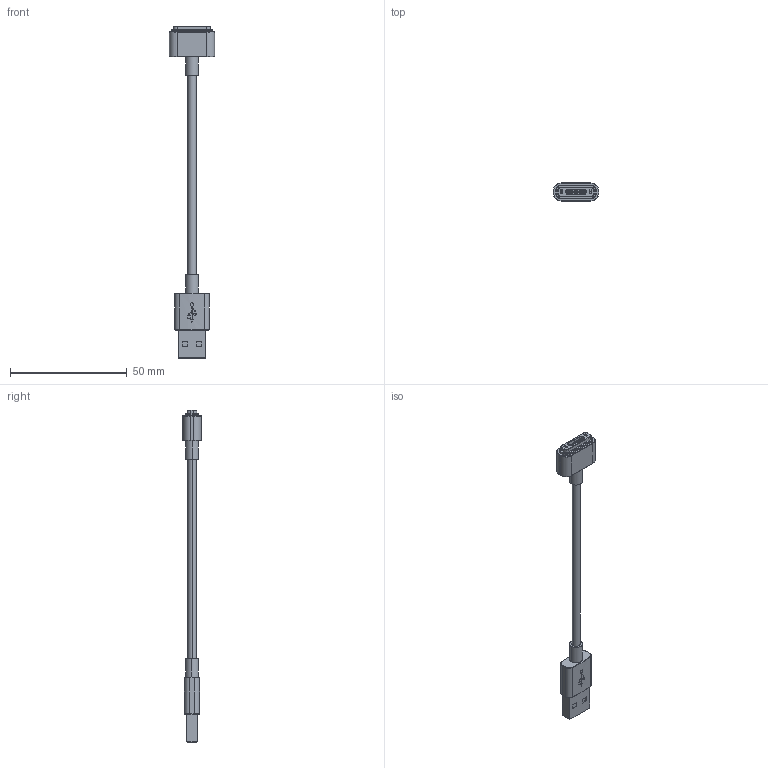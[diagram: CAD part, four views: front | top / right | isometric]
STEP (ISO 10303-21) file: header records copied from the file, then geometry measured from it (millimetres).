
FILE_DESCRIPTION (( 'STEP AP203' ), '1' );
FILE_NAME ('687-G0524A50110E.STEP', '2023-02-14T14:06:00', ( 'Magnum' ), ( '' ), 'SwSTEP 2.0', 'SolidWorks 2020', '' );
FILE_SCHEMA (( 'CONFIG_CONTROL_DESIGN' ));
Length unit declared in the file: millimetre
Products named in the file (1): 687-G0524A50110E
Bounding box: 19.4 x 7.8 x 142.41 mm (x, y, z)
Volume: 4706.2 mm3; surface area: 3668.9 mm2
Topology: 1 solids, 1 shells, 245 faces, 611 edges, 382 vertices
Faces by surface type: plane 101, cylinder 75, torus 41, bspline 18, sphere 10
Entity records: 8317 total; most frequent: CARTESIAN_POINT 2416, DIRECTION 1228, ORIENTED_EDGE 1202, EDGE_CURVE 601, AXIS2_PLACEMENT_3D 458, VERTEX_POINT 382, LINE 312, VECTOR 312
